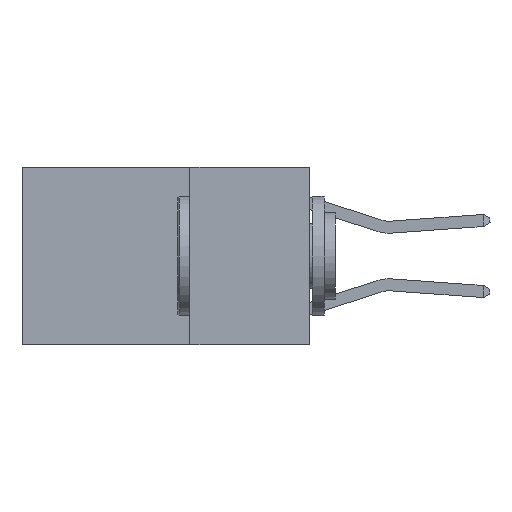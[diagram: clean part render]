
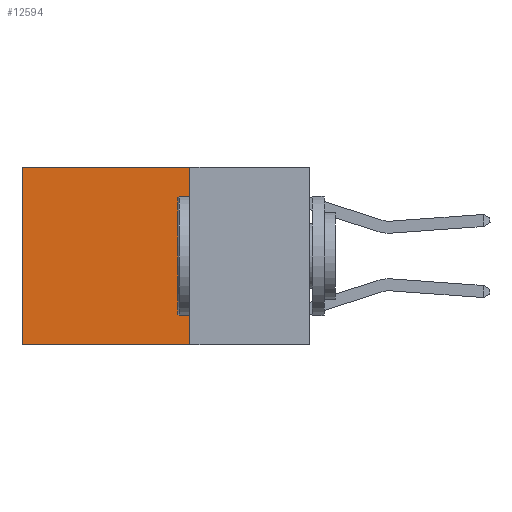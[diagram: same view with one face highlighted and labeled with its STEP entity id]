
A CAD part, left-side view. The second image highlights one B-rep face of the part: STEP entity #12594.
In plain terms, the highlighted planar face has unit normal (-1, 0, 0).
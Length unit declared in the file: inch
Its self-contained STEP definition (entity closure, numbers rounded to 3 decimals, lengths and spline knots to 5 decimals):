
#195 = EDGE_CURVE ( 'NONE', #26472, #16468, #26532, .T. ) ;
#1276 = LINE ( 'NONE', #27161, #3591 ) ;
#3243 = VERTEX_POINT ( 'NONE', #16147 ) ;
#3591 = VECTOR ( 'NONE', #11963, 39.37008 ) ;
#4130 = ORIENTED_EDGE ( 'NONE', *, *, #195, .T. ) ;
#4388 = DIRECTION ( 'NONE',  ( 0., 0., -1. ) ) ;
#4933 = EDGE_CURVE ( 'NONE', #13311, #26472, #20964, .T. ) ;
#5039 = CARTESIAN_POINT ( 'NONE',  ( 0.2625, 0.6, 0. ) ) ;
#5105 = EDGE_CURVE ( 'NONE', #13311, #3243, #1276, .T. ) ;
#7932 = VECTOR ( 'NONE', #15754, 39.37008 ) ;
#8302 = LINE ( 'NONE', #16428, #15164 ) ;
#8849 = AXIS2_PLACEMENT_3D ( 'NONE', #13085, #17071, #4388 ) ;
#10179 = CARTESIAN_POINT ( 'NONE',  ( 0.2625, 0.25, 0. ) ) ;
#11708 = ORIENTED_EDGE ( 'NONE', *, *, #4933, .T. ) ;
#11786 = VECTOR ( 'NONE', #18831, 39.37008 ) ;
#11963 = DIRECTION ( 'NONE',  ( 0., 0., -1. ) ) ;
#12097 = CARTESIAN_POINT ( 'NONE',  ( 0.2625, 0.6, 0. ) ) ;
#12433 = DIRECTION ( 'NONE',  ( 0., 1., 0. ) ) ;
#12594 = ADVANCED_FACE ( 'NONE', ( #16782 ), #12803, .F. ) ;
#12803 = PLANE ( 'NONE',  #8849 ) ;
#13085 = CARTESIAN_POINT ( 'NONE',  ( 0.2625, 0.25, 0. ) ) ;
#13259 = EDGE_CURVE ( 'NONE', #3243, #16468, #8302, .T. ) ;
#13311 = VERTEX_POINT ( 'NONE', #18677 ) ;
#15164 = VECTOR ( 'NONE', #12433, 39.37008 ) ;
#15754 = DIRECTION ( 'NONE',  ( 0., 0., -1. ) ) ;
#16147 = CARTESIAN_POINT ( 'NONE',  ( 0.2625, 0.25, -0.37 ) ) ;
#16417 = ORIENTED_EDGE ( 'NONE', *, *, #13259, .F. ) ;
#16428 = CARTESIAN_POINT ( 'NONE',  ( 0.2625, 0.25, -0.37 ) ) ;
#16468 = VERTEX_POINT ( 'NONE', #22633 ) ;
#16782 = FACE_OUTER_BOUND ( 'NONE', #20615, .T. ) ;
#17071 = DIRECTION ( 'NONE',  ( 1., 0., 0. ) ) ;
#18677 = CARTESIAN_POINT ( 'NONE',  ( 0.2625, 0.25, 0. ) ) ;
#18831 = DIRECTION ( 'NONE',  ( 0., 1., 0. ) ) ;
#20615 = EDGE_LOOP ( 'NONE', ( #4130, #16417, #26071, #11708 ) ) ;
#20964 = LINE ( 'NONE', #10179, #11786 ) ;
#22633 = CARTESIAN_POINT ( 'NONE',  ( 0.2625, 0.6, -0.37 ) ) ;
#26071 = ORIENTED_EDGE ( 'NONE', *, *, #5105, .F. ) ;
#26472 = VERTEX_POINT ( 'NONE', #12097 ) ;
#26532 = LINE ( 'NONE', #5039, #7932 ) ;
#27161 = CARTESIAN_POINT ( 'NONE',  ( 0.2625, 0.25, 0. ) ) ;
